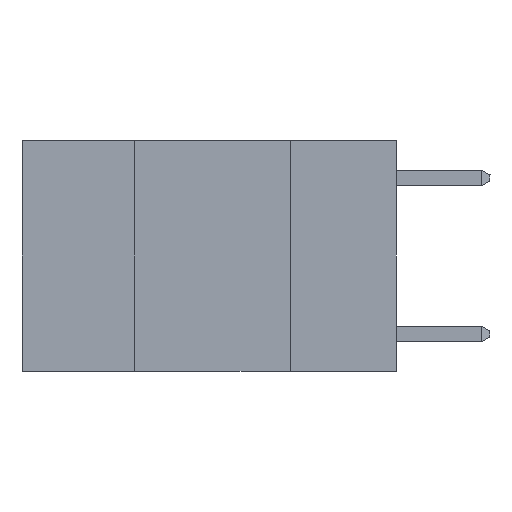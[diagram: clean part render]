
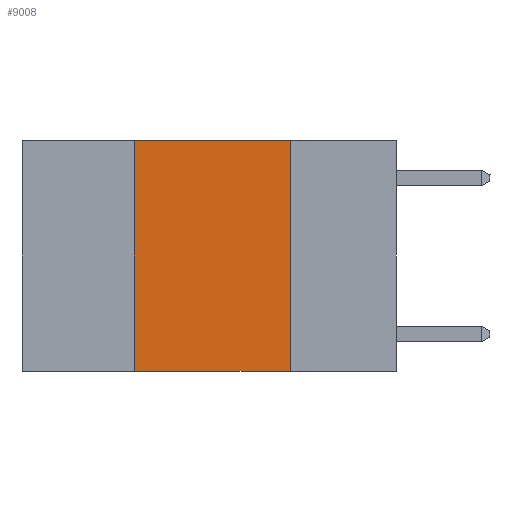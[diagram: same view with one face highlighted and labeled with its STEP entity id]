
A CAD part, left-side view. The second image highlights one B-rep face of the part: STEP entity #9008.
In plain terms, the highlighted planar face has unit normal (-1, 0, 0).
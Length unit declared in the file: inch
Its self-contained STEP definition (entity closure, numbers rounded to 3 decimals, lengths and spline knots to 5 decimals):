
#14 = LINE ( 'NONE', #3137, #2148 ) ;
#934 = EDGE_CURVE ( 'NONE', #8608, #5038, #14, .T. ) ;
#1284 = CARTESIAN_POINT ( 'NONE',  ( 0., 0.6, 0. ) ) ;
#1462 = LINE ( 'NONE', #9278, #7572 ) ;
#2148 = VECTOR ( 'NONE', #6047, 39.37008 ) ;
#2348 = DIRECTION ( 'NONE',  ( 0., 0., -1. ) ) ;
#2416 = CARTESIAN_POINT ( 'NONE',  ( 0., 0.42, -0.37 ) ) ;
#2503 = ORIENTED_EDGE ( 'NONE', *, *, #3952, .F. ) ;
#2565 = VECTOR ( 'NONE', #7516, 39.37008 ) ;
#2763 = CARTESIAN_POINT ( 'NONE',  ( 0., 0.17, 0. ) ) ;
#2829 = PLANE ( 'NONE',  #3997 ) ;
#3137 = CARTESIAN_POINT ( 'NONE',  ( 0., 0.42, 0. ) ) ;
#3685 = VECTOR ( 'NONE', #8590, 39.37008 ) ;
#3697 = DIRECTION ( 'NONE',  ( 0., 0., -1. ) ) ;
#3952 = EDGE_CURVE ( 'NONE', #8438, #6391, #1462, .T. ) ;
#3997 = AXIS2_PLACEMENT_3D ( 'NONE', #1284, #4439, #3697 ) ;
#4173 = LINE ( 'NONE', #6494, #3685 ) ;
#4205 = ORIENTED_EDGE ( 'NONE', *, *, #9553, .F. ) ;
#4439 = DIRECTION ( 'NONE',  ( 1., 0., 0. ) ) ;
#4744 = CARTESIAN_POINT ( 'NONE',  ( 0., 0.17, -0.37 ) ) ;
#5038 = VERTEX_POINT ( 'NONE', #9117 ) ;
#5052 = ORIENTED_EDGE ( 'NONE', *, *, #8674, .T. ) ;
#5162 = LINE ( 'NONE', #9617, #2565 ) ;
#5207 = FACE_OUTER_BOUND ( 'NONE', #7625, .T. ) ;
#6047 = DIRECTION ( 'NONE',  ( 0., 0., 1. ) ) ;
#6170 = ORIENTED_EDGE ( 'NONE', *, *, #934, .F. ) ;
#6391 = VERTEX_POINT ( 'NONE', #4744 ) ;
#6494 = CARTESIAN_POINT ( 'NONE',  ( 0., 0.6, -0.37 ) ) ;
#7516 = DIRECTION ( 'NONE',  ( 0., -1., 0. ) ) ;
#7572 = VECTOR ( 'NONE', #2348, 39.37008 ) ;
#7625 = EDGE_LOOP ( 'NONE', ( #2503, #4205, #6170, #5052 ) ) ;
#8438 = VERTEX_POINT ( 'NONE', #2763 ) ;
#8590 = DIRECTION ( 'NONE',  ( 0., -1., 0. ) ) ;
#8608 = VERTEX_POINT ( 'NONE', #2416 ) ;
#8674 = EDGE_CURVE ( 'NONE', #8608, #6391, #4173, .T. ) ;
#9008 = ADVANCED_FACE ( 'NONE', ( #5207 ), #2829, .F. ) ;
#9117 = CARTESIAN_POINT ( 'NONE',  ( 0., 0.42, 0. ) ) ;
#9278 = CARTESIAN_POINT ( 'NONE',  ( 0., 0.17, 0. ) ) ;
#9553 = EDGE_CURVE ( 'NONE', #5038, #8438, #5162, .T. ) ;
#9617 = CARTESIAN_POINT ( 'NONE',  ( 0., 0.6, 0. ) ) ;
